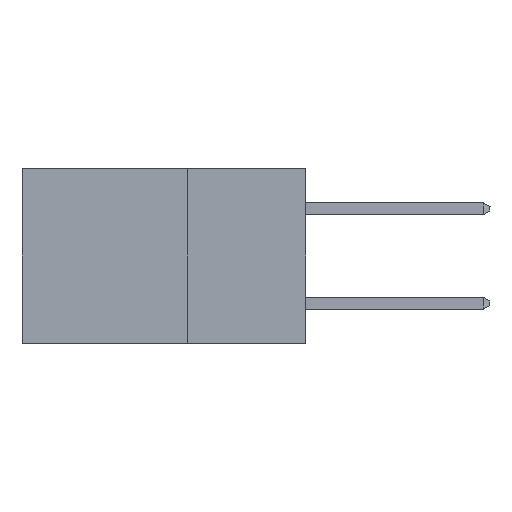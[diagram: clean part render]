
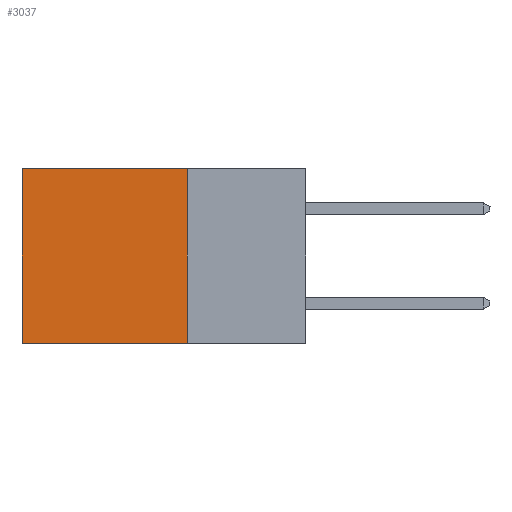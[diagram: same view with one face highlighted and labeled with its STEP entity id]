
A CAD part, left-side view. The second image highlights one B-rep face of the part: STEP entity #3037.
In plain terms, the highlighted planar face has unit normal (-1, 0, 0).
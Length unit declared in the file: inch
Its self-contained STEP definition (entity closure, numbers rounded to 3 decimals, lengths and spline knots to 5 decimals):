
#293 = CARTESIAN_POINT ( 'NONE',  ( 0.298, 0.25, -0.37 ) ) ;
#667 = VECTOR ( 'NONE', #10637, 39.37008 ) ;
#926 = VERTEX_POINT ( 'NONE', #5084 ) ;
#1307 = EDGE_CURVE ( 'NONE', #926, #11663, #19730, .T. ) ;
#3037 = ADVANCED_FACE ( 'NONE', ( #6206 ), #17557, .F. ) ;
#3329 = EDGE_CURVE ( 'NONE', #11663, #27308, #21424, .T. ) ;
#5084 = CARTESIAN_POINT ( 'NONE',  ( 0.298, 0.25, 0. ) ) ;
#6206 = FACE_OUTER_BOUND ( 'NONE', #21558, .T. ) ;
#6884 = VECTOR ( 'NONE', #11827, 39.37008 ) ;
#7977 = ORIENTED_EDGE ( 'NONE', *, *, #11914, .T. ) ;
#8137 = VECTOR ( 'NONE', #14528, 39.37008 ) ;
#10120 = CARTESIAN_POINT ( 'NONE',  ( 0.298, 0.6, -0.37 ) ) ;
#10637 = DIRECTION ( 'NONE',  ( 0., 0., -1. ) ) ;
#11229 = DIRECTION ( 'NONE',  ( 0., 1., 0. ) ) ;
#11663 = VERTEX_POINT ( 'NONE', #293 ) ;
#11827 = DIRECTION ( 'NONE',  ( 0., 1., 0. ) ) ;
#11914 = EDGE_CURVE ( 'NONE', #926, #25581, #29506, .T. ) ;
#14154 = CARTESIAN_POINT ( 'NONE',  ( 0.298, 0.6, 0. ) ) ;
#14498 = EDGE_CURVE ( 'NONE', #25581, #27308, #24216, .T. ) ;
#14528 = DIRECTION ( 'NONE',  ( 0., 0., -1. ) ) ;
#14897 = CARTESIAN_POINT ( 'NONE',  ( 0.298, 0.6, 0. ) ) ;
#15375 = DIRECTION ( 'NONE',  ( 0., 0., -1. ) ) ;
#16055 = VECTOR ( 'NONE', #11229, 39.37008 ) ;
#17557 = PLANE ( 'NONE',  #26656 ) ;
#19229 = CARTESIAN_POINT ( 'NONE',  ( 0.298, 0.25, 0. ) ) ;
#19730 = LINE ( 'NONE', #19229, #8137 ) ;
#21424 = LINE ( 'NONE', #25599, #6884 ) ;
#21503 = ORIENTED_EDGE ( 'NONE', *, *, #14498, .T. ) ;
#21558 = EDGE_LOOP ( 'NONE', ( #21503, #21863, #26785, #7977 ) ) ;
#21863 = ORIENTED_EDGE ( 'NONE', *, *, #3329, .F. ) ;
#22245 = CARTESIAN_POINT ( 'NONE',  ( 0.298, 0.25, 0. ) ) ;
#24216 = LINE ( 'NONE', #14897, #667 ) ;
#25312 = CARTESIAN_POINT ( 'NONE',  ( 0.298, 0.25, 0. ) ) ;
#25581 = VERTEX_POINT ( 'NONE', #14154 ) ;
#25599 = CARTESIAN_POINT ( 'NONE',  ( 0.298, 0.25, -0.37 ) ) ;
#26656 = AXIS2_PLACEMENT_3D ( 'NONE', #22245, #26961, #15375 ) ;
#26785 = ORIENTED_EDGE ( 'NONE', *, *, #1307, .F. ) ;
#26961 = DIRECTION ( 'NONE',  ( 1., 0., 0. ) ) ;
#27308 = VERTEX_POINT ( 'NONE', #10120 ) ;
#29506 = LINE ( 'NONE', #25312, #16055 ) ;
